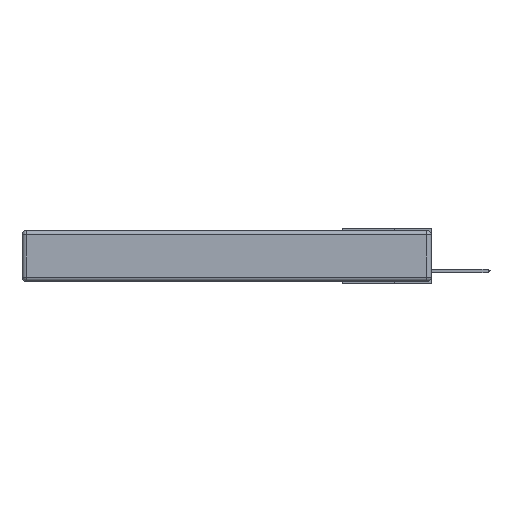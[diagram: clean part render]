
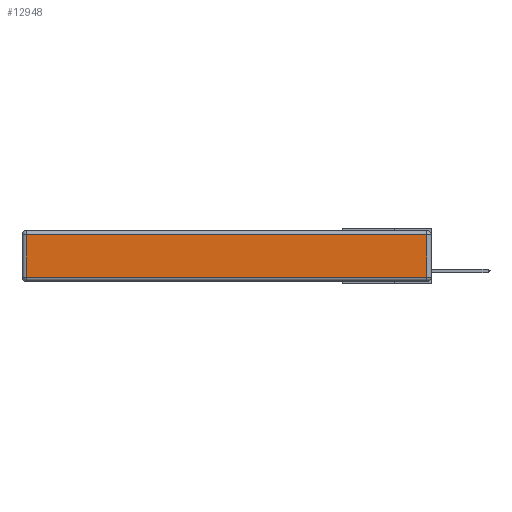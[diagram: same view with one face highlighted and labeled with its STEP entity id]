
A CAD part, left-side view. The second image highlights one B-rep face of the part: STEP entity #12948.
In plain terms, the highlighted planar face has unit normal (-1, 0, 0).
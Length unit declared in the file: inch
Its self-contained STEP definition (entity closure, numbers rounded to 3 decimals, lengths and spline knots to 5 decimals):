
#101 = LINE ( 'NONE', #3795, #5744 ) ;
#273 = DIRECTION ( 'NONE',  ( 0., 0., 1. ) ) ;
#326 = CARTESIAN_POINT ( 'NONE',  ( 0., 0.03, -0.343 ) ) ;
#746 = VECTOR ( 'NONE', #13949, 39.37008 ) ;
#1423 = EDGE_CURVE ( 'NONE', #7496, #13294, #11910, .T. ) ;
#1770 = DIRECTION ( 'NONE',  ( 0., 0., -1. ) ) ;
#1786 = ORIENTED_EDGE ( 'NONE', *, *, #9729, .T. ) ;
#2933 = CARTESIAN_POINT ( 'NONE',  ( 0., 0., -0.313 ) ) ;
#2948 = ORIENTED_EDGE ( 'NONE', *, *, #5765, .T. ) ;
#3677 = CARTESIAN_POINT ( 'NONE',  ( 0., 0.03, -0.313 ) ) ;
#3795 = CARTESIAN_POINT ( 'NONE',  ( 0., 2.72, -0.343 ) ) ;
#4190 = ORIENTED_EDGE ( 'NONE', *, *, #6556, .T. ) ;
#4544 = DIRECTION ( 'NONE',  ( -1., 0., 0. ) ) ;
#4593 = CARTESIAN_POINT ( 'NONE',  ( 0., 0., -0.343 ) ) ;
#4927 = CARTESIAN_POINT ( 'NONE',  ( 0., 0.03, -0.03 ) ) ;
#5035 = VECTOR ( 'NONE', #273, 39.37008 ) ;
#5109 = AXIS2_PLACEMENT_3D ( 'NONE', #4593, #4544, #12526 ) ;
#5736 = VECTOR ( 'NONE', #12196, 39.37008 ) ;
#5744 = VECTOR ( 'NONE', #1770, 39.37008 ) ;
#5765 = EDGE_CURVE ( 'NONE', #13294, #12850, #6829, .T. ) ;
#6556 = EDGE_CURVE ( 'NONE', #9703, #7496, #101, .T. ) ;
#6829 = LINE ( 'NONE', #326, #5035 ) ;
#7249 = LINE ( 'NONE', #11640, #746 ) ;
#7303 = EDGE_LOOP ( 'NONE', ( #10871, #2948, #1786, #4190 ) ) ;
#7496 = VERTEX_POINT ( 'NONE', #13826 ) ;
#9205 = PLANE ( 'NONE',  #5109 ) ;
#9703 = VERTEX_POINT ( 'NONE', #11349 ) ;
#9729 = EDGE_CURVE ( 'NONE', #12850, #9703, #7249, .T. ) ;
#10871 = ORIENTED_EDGE ( 'NONE', *, *, #1423, .T. ) ;
#11349 = CARTESIAN_POINT ( 'NONE',  ( 0., 2.72, -0.03 ) ) ;
#11640 = CARTESIAN_POINT ( 'NONE',  ( 0., 2.75, -0.03 ) ) ;
#11910 = LINE ( 'NONE', #2933, #5736 ) ;
#12196 = DIRECTION ( 'NONE',  ( 0., -1., 0. ) ) ;
#12526 = DIRECTION ( 'NONE',  ( 0., 0., 1. ) ) ;
#12850 = VERTEX_POINT ( 'NONE', #4927 ) ;
#12948 = ADVANCED_FACE ( 'NONE', ( #14836 ), #9205, .T. ) ;
#13294 = VERTEX_POINT ( 'NONE', #3677 ) ;
#13826 = CARTESIAN_POINT ( 'NONE',  ( 0., 2.72, -0.313 ) ) ;
#13949 = DIRECTION ( 'NONE',  ( 0., 1., 0. ) ) ;
#14836 = FACE_OUTER_BOUND ( 'NONE', #7303, .T. ) ;
